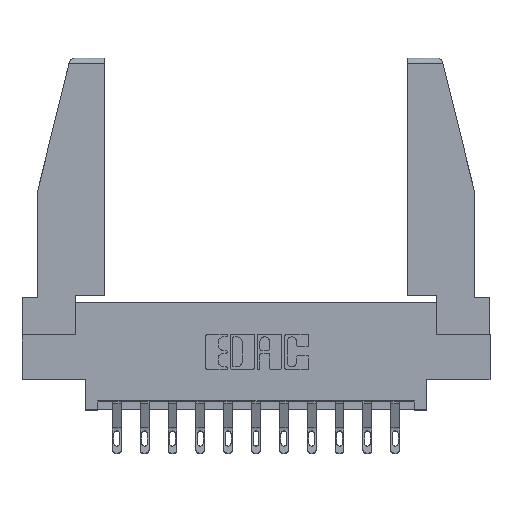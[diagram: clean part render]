
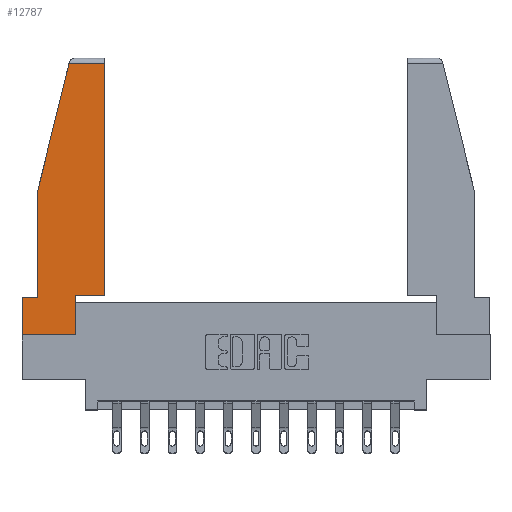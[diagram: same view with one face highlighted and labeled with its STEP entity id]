
A CAD part, top view. The second image highlights one B-rep face of the part: STEP entity #12787.
In plain terms, the highlighted planar face has unit normal (0, 0, 1).
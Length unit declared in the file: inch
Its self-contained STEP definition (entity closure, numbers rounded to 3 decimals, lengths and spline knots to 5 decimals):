
#269 = VERTEX_POINT ( 'NONE', #8355 ) ;
#456 = EDGE_CURVE ( 'NONE', #15121, #269, #2233, .T. ) ;
#535 = LINE ( 'NONE', #4049, #9900 ) ;
#816 = ORIENTED_EDGE ( 'NONE', *, *, #11746, .T. ) ;
#1069 = DIRECTION ( 'NONE',  ( -1., 0., 0. ) ) ;
#1113 = CARTESIAN_POINT ( 'NONE',  ( 0., 1.52, 0. ) ) ;
#1134 = ORIENTED_EDGE ( 'NONE', *, *, #14504, .T. ) ;
#1514 = VERTEX_POINT ( 'NONE', #12145 ) ;
#1648 = CARTESIAN_POINT ( 'NONE',  ( 0., 0., 0. ) ) ;
#1993 = DIRECTION ( 'NONE',  ( 0., -1., 0. ) ) ;
#2029 = EDGE_CURVE ( 'NONE', #2092, #1514, #4411, .T. ) ;
#2092 = VERTEX_POINT ( 'NONE', #7247 ) ;
#2233 = LINE ( 'NONE', #7531, #5429 ) ;
#2343 = VECTOR ( 'NONE', #10753, 39.37008 ) ;
#2497 = EDGE_CURVE ( 'NONE', #7583, #3797, #2510, .T. ) ;
#2504 = CARTESIAN_POINT ( 'NONE',  ( 0.297, 0.223, 0. ) ) ;
#2510 = LINE ( 'NONE', #3353, #5881 ) ;
#2544 = CARTESIAN_POINT ( 'NONE',  ( 0.2636, 1.52, 0. ) ) ;
#2668 = EDGE_LOOP ( 'NONE', ( #9464, #7175, #6642, #12766, #1134, #6608, #816, #4412, #6393 ) ) ;
#2924 = DIRECTION ( 'NONE',  ( 0., 1., 0. ) ) ;
#3097 = DIRECTION ( 'NONE',  ( 1., 0., 0. ) ) ;
#3273 = VECTOR ( 'NONE', #2924, 39.37008 ) ;
#3353 = CARTESIAN_POINT ( 'NONE',  ( 0.271, 1.55, 0. ) ) ;
#3417 = LINE ( 'NONE', #9197, #10682 ) ;
#3521 = AXIS2_PLACEMENT_3D ( 'NONE', #9971, #14911, #3097 ) ;
#3772 = EDGE_CURVE ( 'NONE', #14606, #11340, #3417, .T. ) ;
#3797 = VERTEX_POINT ( 'NONE', #12673 ) ;
#4049 = CARTESIAN_POINT ( 'NONE',  ( 0., 0., 0. ) ) ;
#4293 = EDGE_CURVE ( 'NONE', #269, #7583, #13828, .T. ) ;
#4411 = LINE ( 'NONE', #11608, #3273 ) ;
#4412 = ORIENTED_EDGE ( 'NONE', *, *, #2029, .T. ) ;
#4416 = LINE ( 'NONE', #8396, #2343 ) ;
#4468 = LINE ( 'NONE', #2504, #5788 ) ;
#4598 = CARTESIAN_POINT ( 'NONE',  ( 0.086, 0.8, 0. ) ) ;
#5429 = VECTOR ( 'NONE', #11210, 39.37008 ) ;
#5788 = VECTOR ( 'NONE', #6229, 39.37008 ) ;
#5881 = VECTOR ( 'NONE', #15093, 39.37008 ) ;
#6229 = DIRECTION ( 'NONE',  ( 1., 0., 0. ) ) ;
#6309 = PLANE ( 'NONE',  #3521 ) ;
#6382 = DIRECTION ( 'NONE',  ( 1., 0., 0. ) ) ;
#6393 = ORIENTED_EDGE ( 'NONE', *, *, #13223, .T. ) ;
#6608 = ORIENTED_EDGE ( 'NONE', *, *, #3772, .T. ) ;
#6642 = ORIENTED_EDGE ( 'NONE', *, *, #2497, .T. ) ;
#7175 = ORIENTED_EDGE ( 'NONE', *, *, #4293, .T. ) ;
#7247 = CARTESIAN_POINT ( 'NONE',  ( 0.297, 0., 0. ) ) ;
#7531 = CARTESIAN_POINT ( 'NONE',  ( 0.461, 0.223, 0. ) ) ;
#7583 = VERTEX_POINT ( 'NONE', #2544 ) ;
#8170 = CARTESIAN_POINT ( 'NONE',  ( 0.086, 0.21, 0. ) ) ;
#8355 = CARTESIAN_POINT ( 'NONE',  ( 0.461, 1.52, 0. ) ) ;
#8396 = CARTESIAN_POINT ( 'NONE',  ( 0., 0.21, 0. ) ) ;
#8804 = FACE_OUTER_BOUND ( 'NONE', #2668, .T. ) ;
#9197 = CARTESIAN_POINT ( 'NONE',  ( 0., 0.21, 0. ) ) ;
#9464 = ORIENTED_EDGE ( 'NONE', *, *, #456, .T. ) ;
#9900 = VECTOR ( 'NONE', #6382, 39.37008 ) ;
#9971 = CARTESIAN_POINT ( 'NONE',  ( 0., 0., 0. ) ) ;
#10682 = VECTOR ( 'NONE', #1993, 39.37008 ) ;
#10753 = DIRECTION ( 'NONE',  ( -1., 0., 0. ) ) ;
#11210 = DIRECTION ( 'NONE',  ( 0., 1., 0. ) ) ;
#11230 = VECTOR ( 'NONE', #1069, 39.37008 ) ;
#11340 = VERTEX_POINT ( 'NONE', #1648 ) ;
#11608 = CARTESIAN_POINT ( 'NONE',  ( 0.297, 0., 0. ) ) ;
#11746 = EDGE_CURVE ( 'NONE', #11340, #2092, #535, .T. ) ;
#12007 = VERTEX_POINT ( 'NONE', #8170 ) ;
#12145 = CARTESIAN_POINT ( 'NONE',  ( 0.297, 0.223, 0. ) ) ;
#12653 = VECTOR ( 'NONE', #15365, 39.37008 ) ;
#12673 = CARTESIAN_POINT ( 'NONE',  ( 0.086, 0.8, 0. ) ) ;
#12766 = ORIENTED_EDGE ( 'NONE', *, *, #14843, .T. ) ;
#12787 = ADVANCED_FACE ( 'NONE', ( #8804 ), #6309, .T. ) ;
#13223 = EDGE_CURVE ( 'NONE', #1514, #15121, #4468, .T. ) ;
#13349 = CARTESIAN_POINT ( 'NONE',  ( 0., 0.21, 0. ) ) ;
#13828 = LINE ( 'NONE', #1113, #11230 ) ;
#14504 = EDGE_CURVE ( 'NONE', #12007, #14606, #4416, .T. ) ;
#14536 = LINE ( 'NONE', #4598, #12653 ) ;
#14606 = VERTEX_POINT ( 'NONE', #13349 ) ;
#14707 = CARTESIAN_POINT ( 'NONE',  ( 0.461, 0.223, 0. ) ) ;
#14843 = EDGE_CURVE ( 'NONE', #3797, #12007, #14536, .T. ) ;
#14911 = DIRECTION ( 'NONE',  ( 0., 0., 1. ) ) ;
#15093 = DIRECTION ( 'NONE',  ( -0.239, -0.971, 0. ) ) ;
#15121 = VERTEX_POINT ( 'NONE', #14707 ) ;
#15365 = DIRECTION ( 'NONE',  ( 0., -1., 0. ) ) ;
